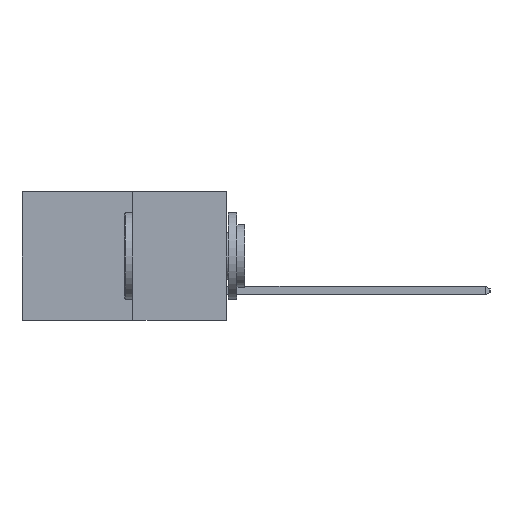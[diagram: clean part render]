
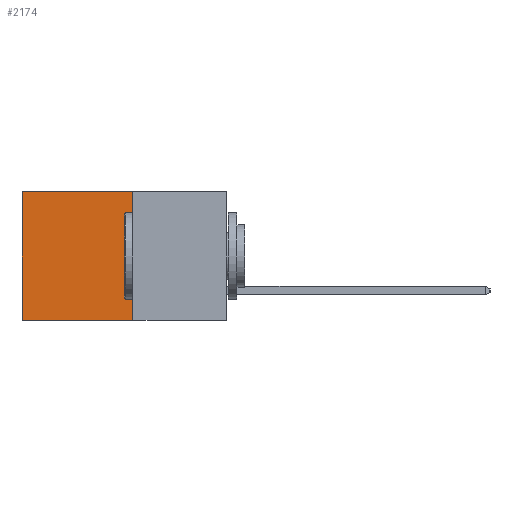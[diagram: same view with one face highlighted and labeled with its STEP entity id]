
A CAD part, left-side view. The second image highlights one B-rep face of the part: STEP entity #2174.
In plain terms, the highlighted planar face has unit normal (-1, 0, 0).
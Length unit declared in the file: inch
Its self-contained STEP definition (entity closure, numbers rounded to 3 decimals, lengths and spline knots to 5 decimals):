
#141 = ORIENTED_EDGE ( 'NONE', *, *, #11155, .F. ) ;
#154 = AXIS2_PLACEMENT_3D ( 'NONE', #9621, #5366, #5231 ) ;
#547 = VERTEX_POINT ( 'NONE', #11468 ) ;
#1568 = VECTOR ( 'NONE', #3629, 39.37008 ) ;
#1582 = FACE_OUTER_BOUND ( 'NONE', #4141, .T. ) ;
#1991 = LINE ( 'NONE', #10364, #6555 ) ;
#2174 = ADVANCED_FACE ( 'NONE', ( #1582 ), #9533, .F. ) ;
#2642 = EDGE_CURVE ( 'NONE', #7592, #10567, #6708, .T. ) ;
#3629 = DIRECTION ( 'NONE',  ( 0., 0., -1. ) ) ;
#4141 = EDGE_LOOP ( 'NONE', ( #9291, #6625, #141, #7183 ) ) ;
#5231 = DIRECTION ( 'NONE',  ( 0., 0., -1. ) ) ;
#5257 = EDGE_CURVE ( 'NONE', #547, #7592, #8968, .T. ) ;
#5366 = DIRECTION ( 'NONE',  ( 1., 0., 0. ) ) ;
#5460 = VECTOR ( 'NONE', #10681, 39.37008 ) ;
#6262 = DIRECTION ( 'NONE',  ( 0., 1., 0. ) ) ;
#6337 = VECTOR ( 'NONE', #6262, 39.37008 ) ;
#6555 = VECTOR ( 'NONE', #11256, 39.37008 ) ;
#6563 = CARTESIAN_POINT ( 'NONE',  ( 0.277, 0.27, 0. ) ) ;
#6625 = ORIENTED_EDGE ( 'NONE', *, *, #6726, .F. ) ;
#6708 = LINE ( 'NONE', #7736, #1568 ) ;
#6726 = EDGE_CURVE ( 'NONE', #6829, #10567, #7825, .T. ) ;
#6829 = VERTEX_POINT ( 'NONE', #8279 ) ;
#7183 = ORIENTED_EDGE ( 'NONE', *, *, #5257, .T. ) ;
#7592 = VERTEX_POINT ( 'NONE', #8366 ) ;
#7736 = CARTESIAN_POINT ( 'NONE',  ( 0.277, 0.59, -0.37 ) ) ;
#7825 = LINE ( 'NONE', #10650, #5460 ) ;
#8279 = CARTESIAN_POINT ( 'NONE',  ( 0.277, 0.27, -0.37 ) ) ;
#8366 = CARTESIAN_POINT ( 'NONE',  ( 0.277, 0.59, 0. ) ) ;
#8968 = LINE ( 'NONE', #6563, #6337 ) ;
#9291 = ORIENTED_EDGE ( 'NONE', *, *, #2642, .T. ) ;
#9533 = PLANE ( 'NONE',  #154 ) ;
#9621 = CARTESIAN_POINT ( 'NONE',  ( 0.277, 0.27, -0.37 ) ) ;
#10364 = CARTESIAN_POINT ( 'NONE',  ( 0.277, 0.27, -0.37 ) ) ;
#10448 = CARTESIAN_POINT ( 'NONE',  ( 0.277, 0.59, -0.37 ) ) ;
#10567 = VERTEX_POINT ( 'NONE', #10448 ) ;
#10650 = CARTESIAN_POINT ( 'NONE',  ( 0.277, 0.27, -0.37 ) ) ;
#10681 = DIRECTION ( 'NONE',  ( 0., 1., 0. ) ) ;
#11155 = EDGE_CURVE ( 'NONE', #547, #6829, #1991, .T. ) ;
#11256 = DIRECTION ( 'NONE',  ( 0., 0., -1. ) ) ;
#11468 = CARTESIAN_POINT ( 'NONE',  ( 0.277, 0.27, 0. ) ) ;
